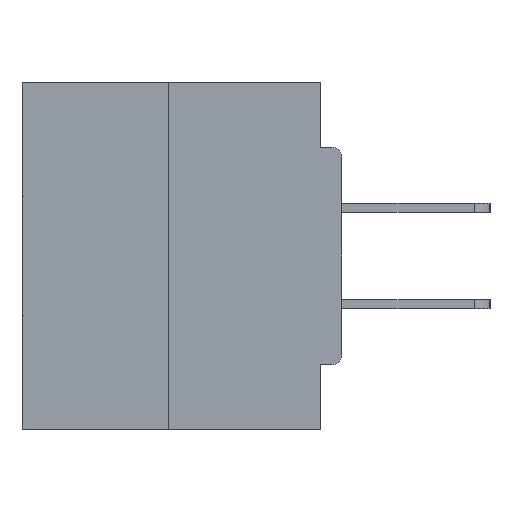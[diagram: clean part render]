
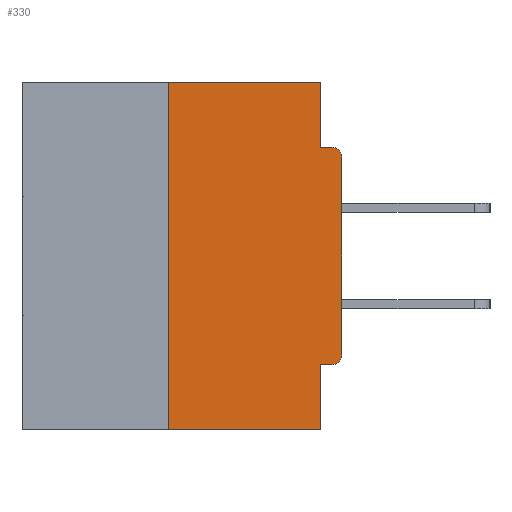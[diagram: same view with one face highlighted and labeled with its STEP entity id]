
A CAD part, left-side view. The second image highlights one B-rep face of the part: STEP entity #330.
In plain terms, the highlighted planar face has unit normal (-1, 0, 0).
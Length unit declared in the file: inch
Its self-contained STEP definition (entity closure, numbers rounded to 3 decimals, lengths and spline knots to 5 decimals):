
#330 = ADVANCED_FACE ( 'NONE', ( #22951 ), #8328, .F. ) ;
#1535 = DIRECTION ( 'NONE',  ( 0., -1., 0. ) ) ;
#1721 = EDGE_CURVE ( 'NONE', #32480, #22488, #13039, .T. ) ;
#1843 = DIRECTION ( 'NONE',  ( 0., -1., 0. ) ) ;
#2027 = ORIENTED_EDGE ( 'NONE', *, *, #2438, .F. ) ;
#2282 = CARTESIAN_POINT ( 'NONE',  ( 0., 0.015, -0.1085 ) ) ;
#2438 = EDGE_CURVE ( 'NONE', #34723, #25843, #29946, .T. ) ;
#3800 = ORIENTED_EDGE ( 'NONE', *, *, #9951, .F. ) ;
#4142 = AXIS2_PLACEMENT_3D ( 'NONE', #2282, #14010, #8813 ) ;
#5159 = VECTOR ( 'NONE', #1535, 39.37008 ) ;
#5543 = DIRECTION ( 'NONE',  ( 0., 1., 0. ) ) ;
#5766 = CIRCLE ( 'NONE', #33510, 0.015 ) ;
#5800 = VECTOR ( 'NONE', #5543, 39.37008 ) ;
#6907 = ORIENTED_EDGE ( 'NONE', *, *, #25233, .F. ) ;
#7568 = ORIENTED_EDGE ( 'NONE', *, *, #21358, .F. ) ;
#8047 = DIRECTION ( 'NONE',  ( 0., 0., 1. ) ) ;
#8243 = CARTESIAN_POINT ( 'NONE',  ( 0., 0.25, 0. ) ) ;
#8328 = PLANE ( 'NONE',  #20363 ) ;
#8518 = ORIENTED_EDGE ( 'NONE', *, *, #16510, .T. ) ;
#8685 = VERTEX_POINT ( 'NONE', #17528 ) ;
#8813 = DIRECTION ( 'NONE',  ( 0., 0., -1. ) ) ;
#9372 = CARTESIAN_POINT ( 'NONE',  ( 0., 0.031, -0.0935 ) ) ;
#9692 = CARTESIAN_POINT ( 'NONE',  ( 0., 0.46, 0. ) ) ;
#9704 = VERTEX_POINT ( 'NONE', #10278 ) ;
#9922 = EDGE_CURVE ( 'NONE', #33538, #28993, #5766, .T. ) ;
#9951 = EDGE_CURVE ( 'NONE', #32751, #8685, #36081, .T. ) ;
#10278 = CARTESIAN_POINT ( 'NONE',  ( 0., 0.25, -0.5 ) ) ;
#10445 = CARTESIAN_POINT ( 'NONE',  ( 0., 0., -0.1085 ) ) ;
#11411 = CARTESIAN_POINT ( 'NONE',  ( 0., 0.015, -0.3915 ) ) ;
#12007 = VECTOR ( 'NONE', #24324, 39.37008 ) ;
#12154 = LINE ( 'NONE', #29332, #22127 ) ;
#13039 = LINE ( 'NONE', #18805, #35005 ) ;
#13348 = DIRECTION ( 'NONE',  ( 1., 0., 0. ) ) ;
#14010 = DIRECTION ( 'NONE',  ( -1., 0., 0. ) ) ;
#14987 = VECTOR ( 'NONE', #15412, 39.37008 ) ;
#15042 = DIRECTION ( 'NONE',  ( 0., 0., -1. ) ) ;
#15412 = DIRECTION ( 'NONE',  ( 0., 0., -1. ) ) ;
#16078 = VERTEX_POINT ( 'NONE', #10445 ) ;
#16412 = ORIENTED_EDGE ( 'NONE', *, *, #9922, .T. ) ;
#16510 = EDGE_CURVE ( 'NONE', #9704, #8685, #27949, .T. ) ;
#17460 = CARTESIAN_POINT ( 'NONE',  ( 0., 0., -0.4065 ) ) ;
#17528 = CARTESIAN_POINT ( 'NONE',  ( 0., 0.031, -0.5 ) ) ;
#18592 = CARTESIAN_POINT ( 'NONE',  ( 0., 0.015, -0.4065 ) ) ;
#18805 = CARTESIAN_POINT ( 'NONE',  ( 0., 0., -0.0935 ) ) ;
#20022 = ORIENTED_EDGE ( 'NONE', *, *, #32272, .F. ) ;
#20051 = CARTESIAN_POINT ( 'NONE',  ( 0., 0.46, 0. ) ) ;
#20149 = LINE ( 'NONE', #17460, #5800 ) ;
#20363 = AXIS2_PLACEMENT_3D ( 'NONE', #20051, #13348, #15042 ) ;
#20396 = CARTESIAN_POINT ( 'NONE',  ( 0., 0.25, 0. ) ) ;
#21026 = CARTESIAN_POINT ( 'NONE',  ( 0., 0., -0.3915 ) ) ;
#21358 = EDGE_CURVE ( 'NONE', #25843, #32480, #30368, .T. ) ;
#21565 = CARTESIAN_POINT ( 'NONE',  ( 0., 0.031, -0.5 ) ) ;
#22127 = VECTOR ( 'NONE', #23881, 39.37008 ) ;
#22488 = VERTEX_POINT ( 'NONE', #25577 ) ;
#22951 = FACE_OUTER_BOUND ( 'NONE', #38059, .T. ) ;
#22955 = VECTOR ( 'NONE', #32673, 39.37008 ) ;
#23881 = DIRECTION ( 'NONE',  ( 0., 0., 1. ) ) ;
#24210 = ORIENTED_EDGE ( 'NONE', *, *, #1721, .F. ) ;
#24324 = DIRECTION ( 'NONE',  ( 0., -1., 0. ) ) ;
#25233 = EDGE_CURVE ( 'NONE', #9704, #34723, #28693, .T. ) ;
#25577 = CARTESIAN_POINT ( 'NONE',  ( 0., 0.015, -0.0935 ) ) ;
#25702 = ORIENTED_EDGE ( 'NONE', *, *, #35157, .T. ) ;
#25843 = VERTEX_POINT ( 'NONE', #32812 ) ;
#26191 = EDGE_CURVE ( 'NONE', #28993, #16078, #12154, .T. ) ;
#26231 = DIRECTION ( 'NONE',  ( -1., 0., 0. ) ) ;
#26698 = CARTESIAN_POINT ( 'NONE',  ( 0., 0.031, 0. ) ) ;
#27383 = CARTESIAN_POINT ( 'NONE',  ( 0., 0.46, -0.5 ) ) ;
#27949 = LINE ( 'NONE', #27383, #5159 ) ;
#28458 = ORIENTED_EDGE ( 'NONE', *, *, #26191, .T. ) ;
#28693 = LINE ( 'NONE', #8243, #30766 ) ;
#28993 = VERTEX_POINT ( 'NONE', #21026 ) ;
#29332 = CARTESIAN_POINT ( 'NONE',  ( 0., 0., 0. ) ) ;
#29946 = LINE ( 'NONE', #9692, #12007 ) ;
#30368 = LINE ( 'NONE', #26698, #22955 ) ;
#30766 = VECTOR ( 'NONE', #8047, 39.37008 ) ;
#32272 = EDGE_CURVE ( 'NONE', #33538, #32751, #20149, .T. ) ;
#32480 = VERTEX_POINT ( 'NONE', #9372 ) ;
#32673 = DIRECTION ( 'NONE',  ( 0., 0., -1. ) ) ;
#32751 = VERTEX_POINT ( 'NONE', #37905 ) ;
#32812 = CARTESIAN_POINT ( 'NONE',  ( 0., 0.031, 0. ) ) ;
#33510 = AXIS2_PLACEMENT_3D ( 'NONE', #11411, #26231, #38014 ) ;
#33538 = VERTEX_POINT ( 'NONE', #18592 ) ;
#34723 = VERTEX_POINT ( 'NONE', #20396 ) ;
#35005 = VECTOR ( 'NONE', #1843, 39.37008 ) ;
#35157 = EDGE_CURVE ( 'NONE', #16078, #22488, #36147, .T. ) ;
#36081 = LINE ( 'NONE', #21565, #14987 ) ;
#36147 = CIRCLE ( 'NONE', #4142, 0.015 ) ;
#37905 = CARTESIAN_POINT ( 'NONE',  ( 0., 0.031, -0.4065 ) ) ;
#38014 = DIRECTION ( 'NONE',  ( 0., 0., -1. ) ) ;
#38059 = EDGE_LOOP ( 'NONE', ( #2027, #6907, #8518, #3800, #20022, #16412, #28458, #25702, #24210, #7568 ) ) ;
